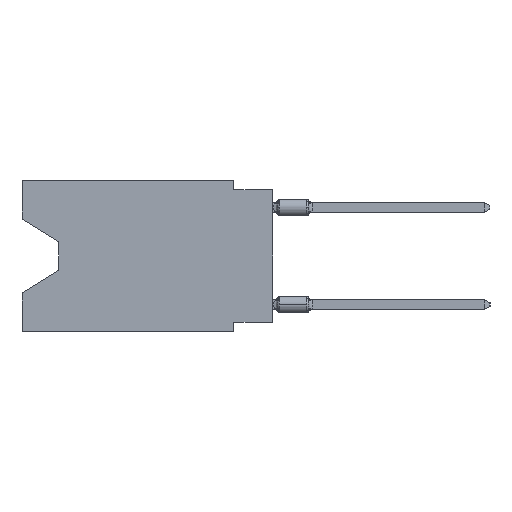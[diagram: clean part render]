
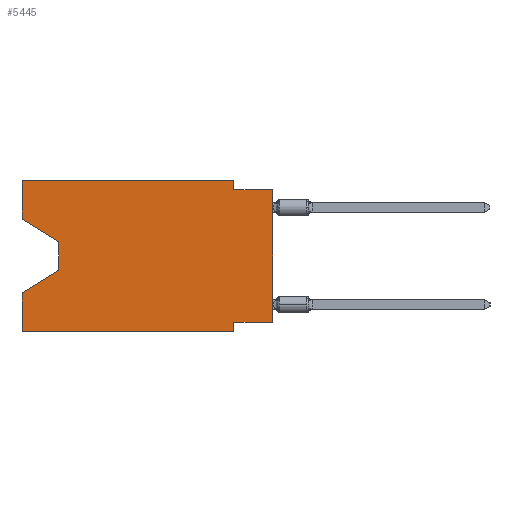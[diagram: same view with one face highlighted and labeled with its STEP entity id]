
A CAD part, left-side view. The second image highlights one B-rep face of the part: STEP entity #5445.
In plain terms, the highlighted planar face has unit normal (-1, 0, 0).
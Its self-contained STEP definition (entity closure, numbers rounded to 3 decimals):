
#3 = CARTESIAN_POINT ( 'NONE',  ( 0., 16.383, -9.906 ) ) ;
#56 = CARTESIAN_POINT ( 'NONE',  ( 0., 0., -9.271 ) ) ;
#1203 = LINE ( 'NONE', #13210, #36182 ) ;
#2444 = EDGE_CURVE ( 'NONE', #32803, #20742, #46478, .T. ) ;
#2597 = EDGE_CURVE ( 'NONE', #32903, #43752, #20970, .T. ) ;
#2925 = ORIENTED_EDGE ( 'NONE', *, *, #11458, .F. ) ;
#3427 = VECTOR ( 'NONE', #36519, 1000. ) ;
#5445 = ADVANCED_FACE ( 'NONE', ( #43028 ), #24521, .F. ) ;
#6599 = VERTEX_POINT ( 'NONE', #20096 ) ;
#7107 = VERTEX_POINT ( 'NONE', #10676 ) ;
#8647 = LINE ( 'NONE', #47360, #27982 ) ;
#9730 = EDGE_CURVE ( 'NONE', #35550, #28916, #40310, .T. ) ;
#10317 = DIRECTION ( 'NONE',  ( 0., -0.855, -0.519 ) ) ;
#10676 = CARTESIAN_POINT ( 'NONE',  ( 0., 2.54, -9.906 ) ) ;
#10745 = CARTESIAN_POINT ( 'NONE',  ( 0., 0., -0.635 ) ) ;
#10898 = EDGE_CURVE ( 'NONE', #13044, #32177, #39088, .T. ) ;
#11324 = VERTEX_POINT ( 'NONE', #21019 ) ;
#11458 = EDGE_CURVE ( 'NONE', #11324, #43752, #48751, .T. ) ;
#12505 = DIRECTION ( 'NONE',  ( 0., 0., -1. ) ) ;
#13006 = CARTESIAN_POINT ( 'NONE',  ( 0., 0., -0.635 ) ) ;
#13044 = VERTEX_POINT ( 'NONE', #36215 ) ;
#13122 = DIRECTION ( 'NONE',  ( 0., 0., 1. ) ) ;
#13210 = CARTESIAN_POINT ( 'NONE',  ( 0., 2.54, -9.906 ) ) ;
#15017 = ORIENTED_EDGE ( 'NONE', *, *, #2444, .T. ) ;
#15182 = ORIENTED_EDGE ( 'NONE', *, *, #10898, .F. ) ;
#15334 = DIRECTION ( 'NONE',  ( 0., 1., 0. ) ) ;
#16382 = ORIENTED_EDGE ( 'NONE', *, *, #36497, .F. ) ;
#16513 = LINE ( 'NONE', #35763, #19545 ) ;
#17420 = ORIENTED_EDGE ( 'NONE', *, *, #2597, .T. ) ;
#17998 = LINE ( 'NONE', #36748, #45042 ) ;
#19132 = ORIENTED_EDGE ( 'NONE', *, *, #9730, .T. ) ;
#19545 = VECTOR ( 'NONE', #12505, 1000. ) ;
#19918 = CARTESIAN_POINT ( 'NONE',  ( 0., 13.97, -5.893 ) ) ;
#20079 = DIRECTION ( 'NONE',  ( 0., 0., -1. ) ) ;
#20096 = CARTESIAN_POINT ( 'NONE',  ( 0., 2.54, -9.271 ) ) ;
#20742 = VERTEX_POINT ( 'NONE', #49253 ) ;
#20970 = LINE ( 'NONE', #25490, #30164 ) ;
#21019 = CARTESIAN_POINT ( 'NONE',  ( 0., 2.54, -0.635 ) ) ;
#21070 = CARTESIAN_POINT ( 'NONE',  ( 0., 2.54, 0. ) ) ;
#23586 = LINE ( 'NONE', #31586, #25421 ) ;
#23675 = LINE ( 'NONE', #31670, #33888 ) ;
#23943 = EDGE_LOOP ( 'NONE', ( #19132, #31095, #15017, #25847, #48683, #25312, #16382, #17420, #2925, #41395, #15182, #45438 ) ) ;
#24521 = PLANE ( 'NONE',  #28839 ) ;
#24625 = EDGE_CURVE ( 'NONE', #6599, #7107, #1203, .T. ) ;
#24838 = DIRECTION ( 'NONE',  ( 0., -1., 0. ) ) ;
#25162 = VECTOR ( 'NONE', #24838, 1000. ) ;
#25312 = ORIENTED_EDGE ( 'NONE', *, *, #24625, .F. ) ;
#25421 = VECTOR ( 'NONE', #20079, 1000. ) ;
#25490 = CARTESIAN_POINT ( 'NONE',  ( 0., 0., 0. ) ) ;
#25847 = ORIENTED_EDGE ( 'NONE', *, *, #28620, .F. ) ;
#26620 = VECTOR ( 'NONE', #10317, 1000. ) ;
#27982 = VECTOR ( 'NONE', #13122, 1000. ) ;
#28533 = DIRECTION ( 'NONE',  ( 1., 0., 0. ) ) ;
#28620 = EDGE_CURVE ( 'NONE', #48657, #20742, #23675, .T. ) ;
#28839 = AXIS2_PLACEMENT_3D ( 'NONE', #31287, #28533, #43757 ) ;
#28916 = VERTEX_POINT ( 'NONE', #33869 ) ;
#29534 = EDGE_CURVE ( 'NONE', #32177, #11324, #16513, .T. ) ;
#30164 = VECTOR ( 'NONE', #40719, 1000. ) ;
#31095 = ORIENTED_EDGE ( 'NONE', *, *, #42120, .T. ) ;
#31287 = CARTESIAN_POINT ( 'NONE',  ( 0., 16.383, 0. ) ) ;
#31533 = VECTOR ( 'NONE', #15334, 1000. ) ;
#31586 = CARTESIAN_POINT ( 'NONE',  ( 0., 13.97, -4.013 ) ) ;
#31670 = CARTESIAN_POINT ( 'NONE',  ( 0., 16.383, 0. ) ) ;
#32177 = VERTEX_POINT ( 'NONE', #21070 ) ;
#32803 = VERTEX_POINT ( 'NONE', #19918 ) ;
#32903 = VERTEX_POINT ( 'NONE', #56 ) ;
#33869 = CARTESIAN_POINT ( 'NONE',  ( 0., 13.97, -4.013 ) ) ;
#33888 = VECTOR ( 'NONE', #39394, 1000. ) ;
#34074 = EDGE_CURVE ( 'NONE', #48657, #7107, #17998, .T. ) ;
#34353 = CARTESIAN_POINT ( 'NONE',  ( 0., 0., -9.271 ) ) ;
#35479 = CARTESIAN_POINT ( 'NONE',  ( 0., 13.97, -5.893 ) ) ;
#35550 = VERTEX_POINT ( 'NONE', #48550 ) ;
#35763 = CARTESIAN_POINT ( 'NONE',  ( 0., 2.54, 0. ) ) ;
#36182 = VECTOR ( 'NONE', #39715, 1000. ) ;
#36215 = CARTESIAN_POINT ( 'NONE',  ( 0., 16.383, 0. ) ) ;
#36240 = DIRECTION ( 'NONE',  ( 0., -1., 0. ) ) ;
#36497 = EDGE_CURVE ( 'NONE', #32903, #6599, #43087, .T. ) ;
#36519 = DIRECTION ( 'NONE',  ( 0., -1., 0. ) ) ;
#36748 = CARTESIAN_POINT ( 'NONE',  ( 0., 16.383, -9.906 ) ) ;
#39088 = LINE ( 'NONE', #47573, #25162 ) ;
#39394 = DIRECTION ( 'NONE',  ( 0., 0., 1. ) ) ;
#39715 = DIRECTION ( 'NONE',  ( 0., 0., -1. ) ) ;
#40310 = LINE ( 'NONE', #48299, #26620 ) ;
#40719 = DIRECTION ( 'NONE',  ( 0., 0., 1. ) ) ;
#41395 = ORIENTED_EDGE ( 'NONE', *, *, #29534, .F. ) ;
#42120 = EDGE_CURVE ( 'NONE', #28916, #32803, #23586, .T. ) ;
#42738 = DIRECTION ( 'NONE',  ( 0., 0.855, -0.519 ) ) ;
#43028 = FACE_OUTER_BOUND ( 'NONE', #23943, .T. ) ;
#43087 = LINE ( 'NONE', #34353, #31533 ) ;
#43752 = VERTEX_POINT ( 'NONE', #13006 ) ;
#43757 = DIRECTION ( 'NONE',  ( 0., 0., -1. ) ) ;
#45042 = VECTOR ( 'NONE', #36240, 1000. ) ;
#45438 = ORIENTED_EDGE ( 'NONE', *, *, #46783, .F. ) ;
#46478 = LINE ( 'NONE', #35479, #48525 ) ;
#46783 = EDGE_CURVE ( 'NONE', #35550, #13044, #8647, .T. ) ;
#47360 = CARTESIAN_POINT ( 'NONE',  ( 0., 16.383, 0. ) ) ;
#47573 = CARTESIAN_POINT ( 'NONE',  ( 0., 16.383, 0. ) ) ;
#48299 = CARTESIAN_POINT ( 'NONE',  ( 0., 16.383, -2.546 ) ) ;
#48525 = VECTOR ( 'NONE', #42738, 1000. ) ;
#48550 = CARTESIAN_POINT ( 'NONE',  ( 0., 16.383, -2.546 ) ) ;
#48657 = VERTEX_POINT ( 'NONE', #3 ) ;
#48683 = ORIENTED_EDGE ( 'NONE', *, *, #34074, .T. ) ;
#48751 = LINE ( 'NONE', #10745, #3427 ) ;
#49253 = CARTESIAN_POINT ( 'NONE',  ( 0., 16.383, -7.36 ) ) ;
